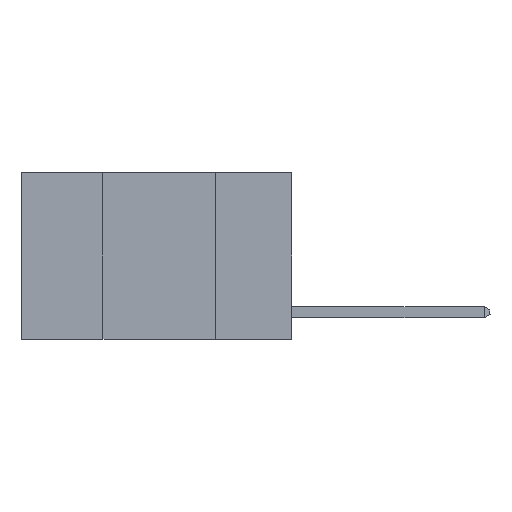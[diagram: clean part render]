
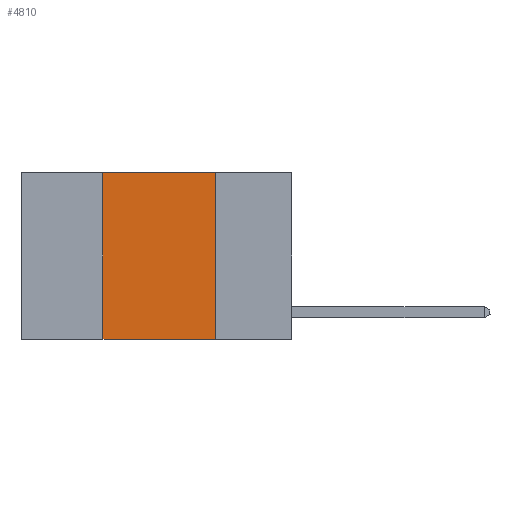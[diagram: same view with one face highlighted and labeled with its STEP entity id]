
A CAD part, left-side view. The second image highlights one B-rep face of the part: STEP entity #4810.
In plain terms, the highlighted planar face has unit normal (-1, 0, 0).
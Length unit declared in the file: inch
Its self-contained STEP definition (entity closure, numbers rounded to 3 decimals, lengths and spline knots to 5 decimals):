
#227 = VERTEX_POINT ( 'NONE', #18473 ) ;
#257 = DIRECTION ( 'NONE',  ( 0., 0., -1. ) ) ;
#488 = VECTOR ( 'NONE', #20462, 39.37008 ) ;
#1306 = VECTOR ( 'NONE', #15356, 39.37008 ) ;
#1777 = ORIENTED_EDGE ( 'NONE', *, *, #19012, .F. ) ;
#1991 = CARTESIAN_POINT ( 'NONE',  ( 0., 0.6, 0. ) ) ;
#2110 = CARTESIAN_POINT ( 'NONE',  ( 0., 0.17, 0. ) ) ;
#2828 = VERTEX_POINT ( 'NONE', #15664 ) ;
#2873 = CARTESIAN_POINT ( 'NONE',  ( 0., 0.6, 0. ) ) ;
#2933 = VERTEX_POINT ( 'NONE', #13361 ) ;
#3967 = AXIS2_PLACEMENT_3D ( 'NONE', #1991, #16015, #257 ) ;
#4099 = VECTOR ( 'NONE', #19111, 39.37008 ) ;
#4810 = ADVANCED_FACE ( 'NONE', ( #21221 ), #5442, .F. ) ;
#5442 = PLANE ( 'NONE',  #3967 ) ;
#6017 = ORIENTED_EDGE ( 'NONE', *, *, #21229, .F. ) ;
#6235 = ORIENTED_EDGE ( 'NONE', *, *, #17104, .T. ) ;
#9939 = EDGE_LOOP ( 'NONE', ( #6017, #1777, #22230, #6235 ) ) ;
#10708 = LINE ( 'NONE', #12350, #4099 ) ;
#11070 = LINE ( 'NONE', #2110, #21080 ) ;
#11838 = VERTEX_POINT ( 'NONE', #16977 ) ;
#12350 = CARTESIAN_POINT ( 'NONE',  ( 0., 0.6, -0.37 ) ) ;
#13361 = CARTESIAN_POINT ( 'NONE',  ( 0., 0.17, 0. ) ) ;
#15250 = LINE ( 'NONE', #19032, #1306 ) ;
#15356 = DIRECTION ( 'NONE',  ( 0., 0., 1. ) ) ;
#15664 = CARTESIAN_POINT ( 'NONE',  ( 0., 0.42, -0.37 ) ) ;
#16015 = DIRECTION ( 'NONE',  ( 1., 0., 0. ) ) ;
#16640 = LINE ( 'NONE', #2873, #488 ) ;
#16977 = CARTESIAN_POINT ( 'NONE',  ( 0., 0.17, -0.37 ) ) ;
#17104 = EDGE_CURVE ( 'NONE', #2828, #11838, #10708, .T. ) ;
#17420 = EDGE_CURVE ( 'NONE', #2828, #227, #15250, .T. ) ;
#18086 = DIRECTION ( 'NONE',  ( 0., 0., -1. ) ) ;
#18473 = CARTESIAN_POINT ( 'NONE',  ( 0., 0.42, 0. ) ) ;
#19012 = EDGE_CURVE ( 'NONE', #227, #2933, #16640, .T. ) ;
#19032 = CARTESIAN_POINT ( 'NONE',  ( 0., 0.42, 0. ) ) ;
#19111 = DIRECTION ( 'NONE',  ( 0., -1., 0. ) ) ;
#20462 = DIRECTION ( 'NONE',  ( 0., -1., 0. ) ) ;
#21080 = VECTOR ( 'NONE', #18086, 39.37008 ) ;
#21221 = FACE_OUTER_BOUND ( 'NONE', #9939, .T. ) ;
#21229 = EDGE_CURVE ( 'NONE', #2933, #11838, #11070, .T. ) ;
#22230 = ORIENTED_EDGE ( 'NONE', *, *, #17420, .F. ) ;
